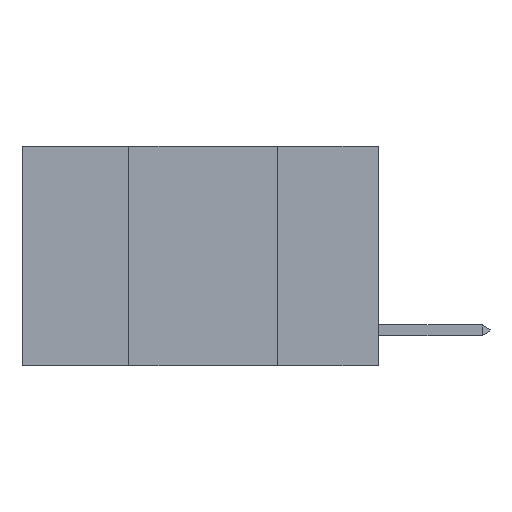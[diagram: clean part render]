
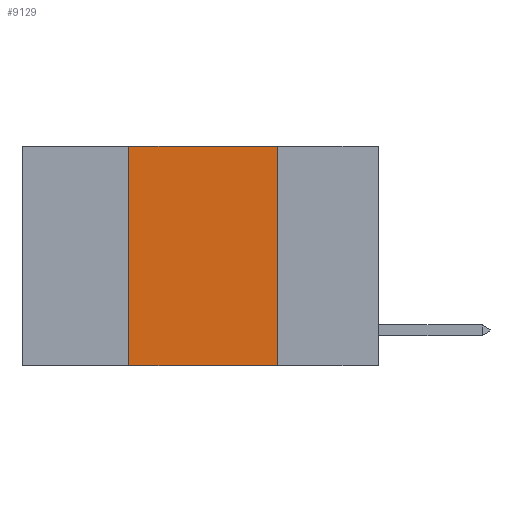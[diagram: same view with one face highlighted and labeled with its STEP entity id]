
A CAD part, left-side view. The second image highlights one B-rep face of the part: STEP entity #9129.
In plain terms, the highlighted planar face has unit normal (-1, 0, 0).
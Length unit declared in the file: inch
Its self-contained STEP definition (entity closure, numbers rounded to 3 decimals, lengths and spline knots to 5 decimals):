
#83 = CARTESIAN_POINT ( 'NONE',  ( 0., 0.17, 0. ) ) ;
#188 = LINE ( 'NONE', #4487, #816 ) ;
#313 = CARTESIAN_POINT ( 'NONE',  ( 0., 0.42, 0. ) ) ;
#403 = DIRECTION ( 'NONE',  ( 1., 0., 0. ) ) ;
#738 = VECTOR ( 'NONE', #8015, 39.37008 ) ;
#816 = VECTOR ( 'NONE', #6073, 39.37008 ) ;
#1009 = DIRECTION ( 'NONE',  ( 0., -1., 0. ) ) ;
#1211 = CARTESIAN_POINT ( 'NONE',  ( 0., 0.17, 0. ) ) ;
#1952 = VERTEX_POINT ( 'NONE', #3673 ) ;
#1980 = EDGE_CURVE ( 'NONE', #1952, #7505, #5217, .T. ) ;
#2519 = CARTESIAN_POINT ( 'NONE',  ( 0., 0.6, 0. ) ) ;
#2754 = ORIENTED_EDGE ( 'NONE', *, *, #8507, .F. ) ;
#2989 = VECTOR ( 'NONE', #4862, 39.37008 ) ;
#3310 = FACE_OUTER_BOUND ( 'NONE', #9024, .T. ) ;
#3393 = PLANE ( 'NONE',  #4164 ) ;
#3673 = CARTESIAN_POINT ( 'NONE',  ( 0., 0.42, -0.37 ) ) ;
#3946 = CARTESIAN_POINT ( 'NONE',  ( 0., 0.17, -0.37 ) ) ;
#4124 = VERTEX_POINT ( 'NONE', #83 ) ;
#4132 = CARTESIAN_POINT ( 'NONE',  ( 0., 0.42, 0. ) ) ;
#4164 = AXIS2_PLACEMENT_3D ( 'NONE', #2519, #403, #7503 ) ;
#4193 = VERTEX_POINT ( 'NONE', #3946 ) ;
#4466 = CARTESIAN_POINT ( 'NONE',  ( 0., 0.6, -0.37 ) ) ;
#4487 = CARTESIAN_POINT ( 'NONE',  ( 0., 0.6, 0. ) ) ;
#4652 = ORIENTED_EDGE ( 'NONE', *, *, #7497, .F. ) ;
#4862 = DIRECTION ( 'NONE',  ( 0., 0., -1. ) ) ;
#5210 = VECTOR ( 'NONE', #1009, 39.37008 ) ;
#5217 = LINE ( 'NONE', #313, #738 ) ;
#6073 = DIRECTION ( 'NONE',  ( 0., -1., 0. ) ) ;
#6162 = LINE ( 'NONE', #1211, #2989 ) ;
#6229 = EDGE_CURVE ( 'NONE', #1952, #4193, #8114, .T. ) ;
#6351 = ORIENTED_EDGE ( 'NONE', *, *, #6229, .T. ) ;
#6696 = ORIENTED_EDGE ( 'NONE', *, *, #1980, .F. ) ;
#7497 = EDGE_CURVE ( 'NONE', #4124, #4193, #6162, .T. ) ;
#7503 = DIRECTION ( 'NONE',  ( 0., 0., -1. ) ) ;
#7505 = VERTEX_POINT ( 'NONE', #4132 ) ;
#8015 = DIRECTION ( 'NONE',  ( 0., 0., 1. ) ) ;
#8114 = LINE ( 'NONE', #4466, #5210 ) ;
#8507 = EDGE_CURVE ( 'NONE', #7505, #4124, #188, .T. ) ;
#9024 = EDGE_LOOP ( 'NONE', ( #4652, #2754, #6696, #6351 ) ) ;
#9129 = ADVANCED_FACE ( 'NONE', ( #3310 ), #3393, .F. ) ;
